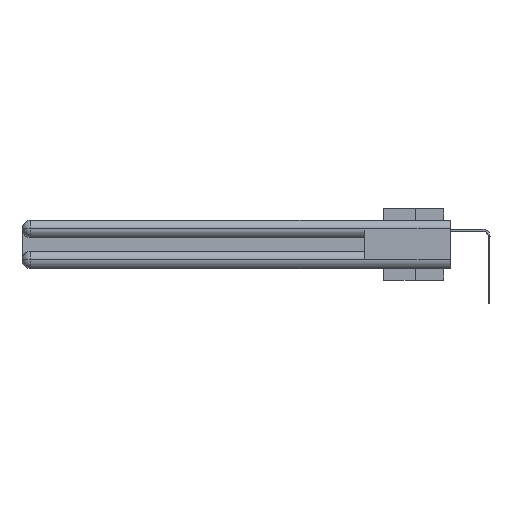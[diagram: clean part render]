
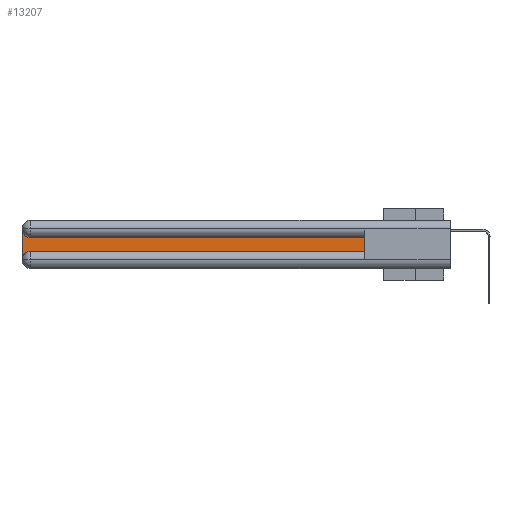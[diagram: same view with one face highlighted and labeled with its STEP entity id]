
A CAD part, left-side view. The second image highlights one B-rep face of the part: STEP entity #13207.
In plain terms, the highlighted planar face has unit normal (-1, 0, 0).
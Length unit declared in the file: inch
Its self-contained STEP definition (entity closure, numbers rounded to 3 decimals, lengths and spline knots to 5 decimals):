
#605 = CARTESIAN_POINT ( 'NONE',  ( 0.075, 3., -0.2175 ) ) ;
#1569 = DIRECTION ( 'NONE',  ( 0., 0., -1. ) ) ;
#1685 = AXIS2_PLACEMENT_3D ( 'NONE', #4253, #9894, #20420 ) ;
#3503 = ORIENTED_EDGE ( 'NONE', *, *, #29060, .T. ) ;
#4217 = CARTESIAN_POINT ( 'NONE',  ( 0.075, 0.6, -0.2175 ) ) ;
#4253 = CARTESIAN_POINT ( 'NONE',  ( 0.075, 3., -0.1225 ) ) ;
#4976 = ORIENTED_EDGE ( 'NONE', *, *, #32059, .T. ) ;
#5068 = CARTESIAN_POINT ( 'NONE',  ( 0.075, 2.94, -0.2775 ) ) ;
#5542 = ORIENTED_EDGE ( 'NONE', *, *, #28842, .T. ) ;
#5873 = EDGE_CURVE ( 'NONE', #30385, #18852, #15673, .T. ) ;
#6211 = VECTOR ( 'NONE', #23273, 39.37008 ) ;
#6514 = CARTESIAN_POINT ( 'NONE',  ( 0.075, 2.94, -0.2175 ) ) ;
#6998 = PLANE ( 'NONE',  #1685 ) ;
#7139 = VERTEX_POINT ( 'NONE', #32720 ) ;
#8137 = DIRECTION ( 'NONE',  ( 0., 1., 0. ) ) ;
#8756 = EDGE_CURVE ( 'NONE', #7139, #30385, #27005, .T. ) ;
#9894 = DIRECTION ( 'NONE',  ( 1., 0., 0. ) ) ;
#10315 = AXIS2_PLACEMENT_3D ( 'NONE', #23665, #15446, #1569 ) ;
#12637 = EDGE_LOOP ( 'NONE', ( #3503, #26318, #13989, #4976, #5542, #22906 ) ) ;
#12798 = DIRECTION ( 'NONE',  ( 0., 0., -1. ) ) ;
#13207 = ADVANCED_FACE ( 'NONE', ( #13996 ), #6998, .F. ) ;
#13607 = VERTEX_POINT ( 'NONE', #4217 ) ;
#13989 = ORIENTED_EDGE ( 'NONE', *, *, #5873, .T. ) ;
#13996 = FACE_OUTER_BOUND ( 'NONE', #12637, .T. ) ;
#15446 = DIRECTION ( 'NONE',  ( 1., 0., 0. ) ) ;
#15673 = LINE ( 'NONE', #605, #18714 ) ;
#16193 = DIRECTION ( 'NONE',  ( 0., 0., 1. ) ) ;
#18714 = VECTOR ( 'NONE', #25110, 39.37008 ) ;
#18852 = VERTEX_POINT ( 'NONE', #28018 ) ;
#20420 = DIRECTION ( 'NONE',  ( 0., 0., -1. ) ) ;
#22862 = LINE ( 'NONE', #32877, #26729 ) ;
#22906 = ORIENTED_EDGE ( 'NONE', *, *, #33406, .T. ) ;
#23273 = DIRECTION ( 'NONE',  ( 0., -1., 0. ) ) ;
#23665 = CARTESIAN_POINT ( 'NONE',  ( 0.075, 2.94, -0.0625 ) ) ;
#25110 = DIRECTION ( 'NONE',  ( 0., 0., -1. ) ) ;
#25148 = VERTEX_POINT ( 'NONE', #6514 ) ;
#26118 = VERTEX_POINT ( 'NONE', #29256 ) ;
#26318 = ORIENTED_EDGE ( 'NONE', *, *, #8756, .T. ) ;
#26729 = VECTOR ( 'NONE', #16193, 39.37008 ) ;
#26806 = DIRECTION ( 'NONE',  ( 1., 0., 0. ) ) ;
#27005 = CIRCLE ( 'NONE', #10315, 0.06 ) ;
#27343 = LINE ( 'NONE', #29196, #32976 ) ;
#28018 = CARTESIAN_POINT ( 'NONE',  ( 0.075, 3., -0.2775 ) ) ;
#28842 = EDGE_CURVE ( 'NONE', #25148, #13607, #33012, .T. ) ;
#29060 = EDGE_CURVE ( 'NONE', #26118, #7139, #27343, .T. ) ;
#29196 = CARTESIAN_POINT ( 'NONE',  ( 0.075, 0.6, -0.1225 ) ) ;
#29256 = CARTESIAN_POINT ( 'NONE',  ( 0.075, 0.6, -0.1225 ) ) ;
#30385 = VERTEX_POINT ( 'NONE', #35775 ) ;
#32059 = EDGE_CURVE ( 'NONE', #18852, #25148, #32828, .T. ) ;
#32720 = CARTESIAN_POINT ( 'NONE',  ( 0.075, 2.94, -0.1225 ) ) ;
#32828 = CIRCLE ( 'NONE', #35454, 0.06 ) ;
#32877 = CARTESIAN_POINT ( 'NONE',  ( 0.075, 0.6, -0.2175 ) ) ;
#32976 = VECTOR ( 'NONE', #8137, 39.37008 ) ;
#33012 = LINE ( 'NONE', #34160, #6211 ) ;
#33406 = EDGE_CURVE ( 'NONE', #13607, #26118, #22862, .T. ) ;
#34160 = CARTESIAN_POINT ( 'NONE',  ( 0.075, 0.6, -0.2175 ) ) ;
#35454 = AXIS2_PLACEMENT_3D ( 'NONE', #5068, #26806, #12798 ) ;
#35775 = CARTESIAN_POINT ( 'NONE',  ( 0.075, 3., -0.0625 ) ) ;
